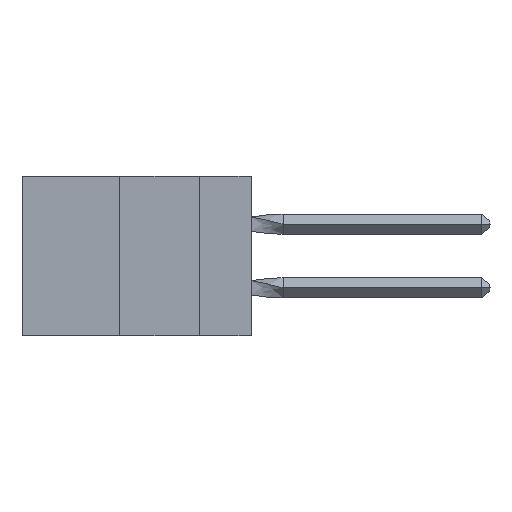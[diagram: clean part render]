
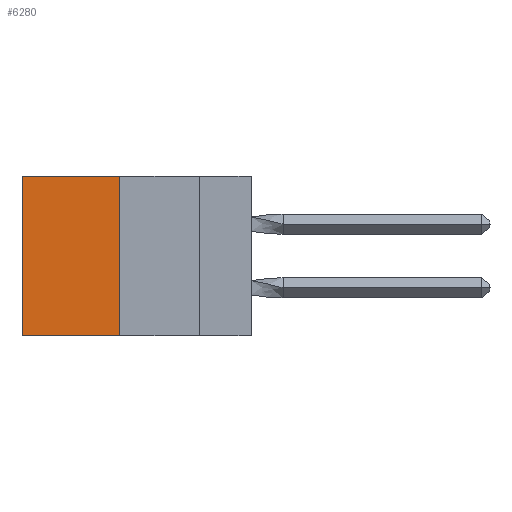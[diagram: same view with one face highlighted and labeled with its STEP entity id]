
A CAD part, left-side view. The second image highlights one B-rep face of the part: STEP entity #6280.
In plain terms, the highlighted planar face has unit normal (-1, 0, 0).
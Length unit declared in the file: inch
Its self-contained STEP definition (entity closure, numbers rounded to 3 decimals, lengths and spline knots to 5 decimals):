
#509 = CARTESIAN_POINT ( 'NONE',  ( 0.305, 0.72, -0.5 ) ) ;
#604 = CARTESIAN_POINT ( 'NONE',  ( 0.305, 0.413, -0.5 ) ) ;
#883 = ORIENTED_EDGE ( 'NONE', *, *, #2343, .F. ) ;
#1401 = LINE ( 'NONE', #21353, #13047 ) ;
#1625 = DIRECTION ( 'NONE',  ( 0., 0., -1. ) ) ;
#2343 = EDGE_CURVE ( 'NONE', #14777, #21419, #18492, .T. ) ;
#3782 = CARTESIAN_POINT ( 'NONE',  ( 0.305, 0.413, -0.5 ) ) ;
#5827 = ORIENTED_EDGE ( 'NONE', *, *, #7131, .F. ) ;
#6280 = ADVANCED_FACE ( 'NONE', ( #7586 ), #16093, .F. ) ;
#7004 = EDGE_CURVE ( 'NONE', #10620, #10718, #15704, .T. ) ;
#7131 = EDGE_CURVE ( 'NONE', #10620, #14777, #1401, .T. ) ;
#7586 = FACE_OUTER_BOUND ( 'NONE', #14592, .T. ) ;
#10620 = VERTEX_POINT ( 'NONE', #15918 ) ;
#10718 = VERTEX_POINT ( 'NONE', #25592 ) ;
#11075 = DIRECTION ( 'NONE',  ( 0., 0., -1. ) ) ;
#11673 = VECTOR ( 'NONE', #18016, 39.37008 ) ;
#11951 = CARTESIAN_POINT ( 'NONE',  ( 0.305, 0.72, -0.5 ) ) ;
#12514 = ORIENTED_EDGE ( 'NONE', *, *, #14803, .T. ) ;
#13047 = VECTOR ( 'NONE', #15113, 39.37008 ) ;
#14480 = DIRECTION ( 'NONE',  ( 0., 1., 0. ) ) ;
#14592 = EDGE_LOOP ( 'NONE', ( #12514, #883, #5827, #21724 ) ) ;
#14777 = VERTEX_POINT ( 'NONE', #604 ) ;
#14803 = EDGE_CURVE ( 'NONE', #10718, #21419, #15267, .T. ) ;
#15113 = DIRECTION ( 'NONE',  ( 0., 0., -1. ) ) ;
#15267 = LINE ( 'NONE', #509, #24620 ) ;
#15704 = LINE ( 'NONE', #22500, #20240 ) ;
#15918 = CARTESIAN_POINT ( 'NONE',  ( 0.305, 0.413, 0. ) ) ;
#16093 = PLANE ( 'NONE',  #16930 ) ;
#16930 = AXIS2_PLACEMENT_3D ( 'NONE', #3782, #18440, #1625 ) ;
#18016 = DIRECTION ( 'NONE',  ( 0., 1., 0. ) ) ;
#18440 = DIRECTION ( 'NONE',  ( 1., 0., 0. ) ) ;
#18492 = LINE ( 'NONE', #19382, #11673 ) ;
#19382 = CARTESIAN_POINT ( 'NONE',  ( 0.305, 0.413, -0.5 ) ) ;
#20240 = VECTOR ( 'NONE', #14480, 39.37008 ) ;
#21353 = CARTESIAN_POINT ( 'NONE',  ( 0.305, 0.413, -0.5 ) ) ;
#21419 = VERTEX_POINT ( 'NONE', #11951 ) ;
#21724 = ORIENTED_EDGE ( 'NONE', *, *, #7004, .T. ) ;
#22500 = CARTESIAN_POINT ( 'NONE',  ( 0.305, 0.413, 0. ) ) ;
#24620 = VECTOR ( 'NONE', #11075, 39.37008 ) ;
#25592 = CARTESIAN_POINT ( 'NONE',  ( 0.305, 0.72, 0. ) ) ;
